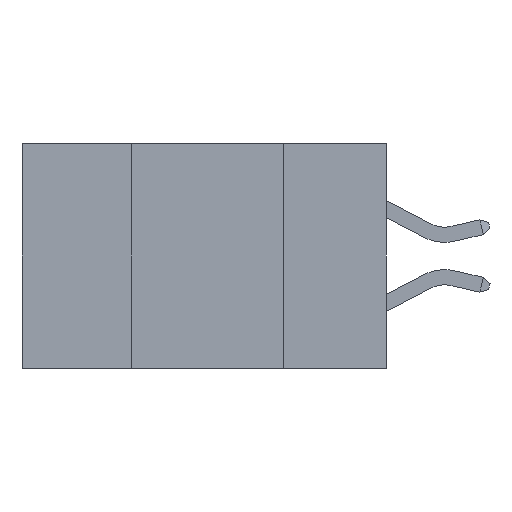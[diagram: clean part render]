
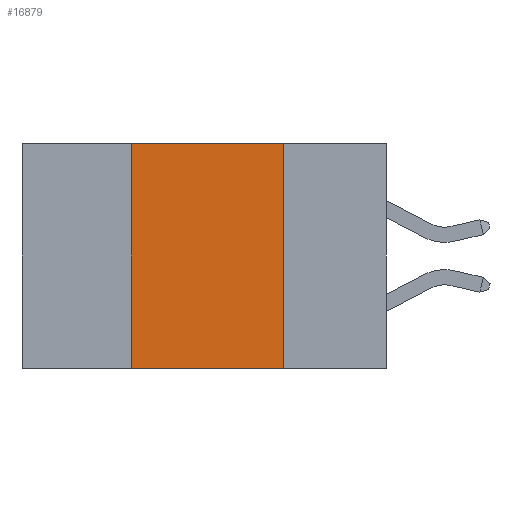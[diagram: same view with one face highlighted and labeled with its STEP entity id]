
A CAD part, left-side view. The second image highlights one B-rep face of the part: STEP entity #16879.
In plain terms, the highlighted planar face has unit normal (-1, 0, 0).
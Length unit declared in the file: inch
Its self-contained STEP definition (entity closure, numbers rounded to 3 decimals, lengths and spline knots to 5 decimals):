
#430 = DIRECTION ( 'NONE',  ( 1., 0., 0. ) ) ;
#1172 = EDGE_LOOP ( 'NONE', ( #17602, #19086, #7334, #21844 ) ) ;
#1178 = LINE ( 'NONE', #10096, #6565 ) ;
#2232 = EDGE_CURVE ( 'NONE', #20474, #19782, #4887, .T. ) ;
#3331 = VERTEX_POINT ( 'NONE', #10326 ) ;
#4148 = CARTESIAN_POINT ( 'NONE',  ( 0., 0.17, 0. ) ) ;
#4758 = EDGE_CURVE ( 'NONE', #19782, #8009, #25986, .T. ) ;
#4768 = LINE ( 'NONE', #5202, #20239 ) ;
#4887 = LINE ( 'NONE', #19609, #25563 ) ;
#5202 = CARTESIAN_POINT ( 'NONE',  ( 0., 0.6, -0.37 ) ) ;
#6468 = CARTESIAN_POINT ( 'NONE',  ( 0., 0.6, 0. ) ) ;
#6565 = VECTOR ( 'NONE', #22107, 39.37008 ) ;
#7212 = DIRECTION ( 'NONE',  ( 0., -1., 0. ) ) ;
#7334 = ORIENTED_EDGE ( 'NONE', *, *, #21789, .F. ) ;
#8009 = VERTEX_POINT ( 'NONE', #23068 ) ;
#8660 = CARTESIAN_POINT ( 'NONE',  ( 0., 0.17, -0.37 ) ) ;
#10096 = CARTESIAN_POINT ( 'NONE',  ( 0., 0.42, -0.37 ) ) ;
#10326 = CARTESIAN_POINT ( 'NONE',  ( 0., 0.42, -0.37 ) ) ;
#10727 = DIRECTION ( 'NONE',  ( 0., 0., -1. ) ) ;
#12623 = PLANE ( 'NONE',  #14847 ) ;
#12978 = FACE_OUTER_BOUND ( 'NONE', #1172, .T. ) ;
#14660 = DIRECTION ( 'NONE',  ( 0., 0., -1. ) ) ;
#14847 = AXIS2_PLACEMENT_3D ( 'NONE', #6468, #430, #14660 ) ;
#16879 = ADVANCED_FACE ( 'NONE', ( #12978 ), #12623, .F. ) ;
#17602 = ORIENTED_EDGE ( 'NONE', *, *, #4758, .F. ) ;
#19086 = ORIENTED_EDGE ( 'NONE', *, *, #2232, .F. ) ;
#19609 = CARTESIAN_POINT ( 'NONE',  ( 0., 0.6, 0. ) ) ;
#19782 = VERTEX_POINT ( 'NONE', #4148 ) ;
#20038 = DIRECTION ( 'NONE',  ( 0., -1., 0. ) ) ;
#20147 = EDGE_CURVE ( 'NONE', #3331, #8009, #4768, .T. ) ;
#20239 = VECTOR ( 'NONE', #7212, 39.37008 ) ;
#20474 = VERTEX_POINT ( 'NONE', #22084 ) ;
#20789 = VECTOR ( 'NONE', #10727, 39.37008 ) ;
#21789 = EDGE_CURVE ( 'NONE', #3331, #20474, #1178, .T. ) ;
#21844 = ORIENTED_EDGE ( 'NONE', *, *, #20147, .T. ) ;
#22084 = CARTESIAN_POINT ( 'NONE',  ( 0., 0.42, 0. ) ) ;
#22107 = DIRECTION ( 'NONE',  ( 0., 0., 1. ) ) ;
#23068 = CARTESIAN_POINT ( 'NONE',  ( 0., 0.17, -0.37 ) ) ;
#25563 = VECTOR ( 'NONE', #20038, 39.37008 ) ;
#25986 = LINE ( 'NONE', #8660, #20789 ) ;
